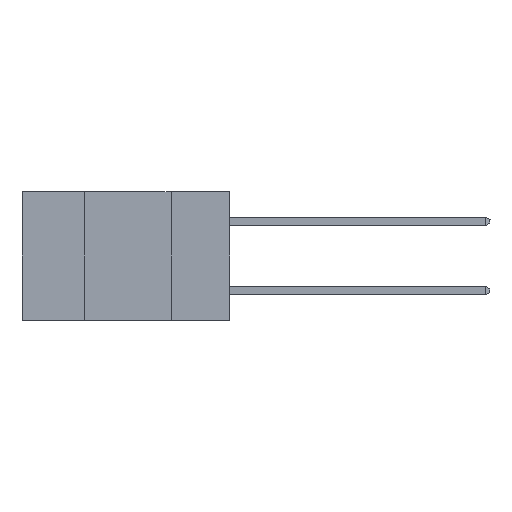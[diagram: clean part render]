
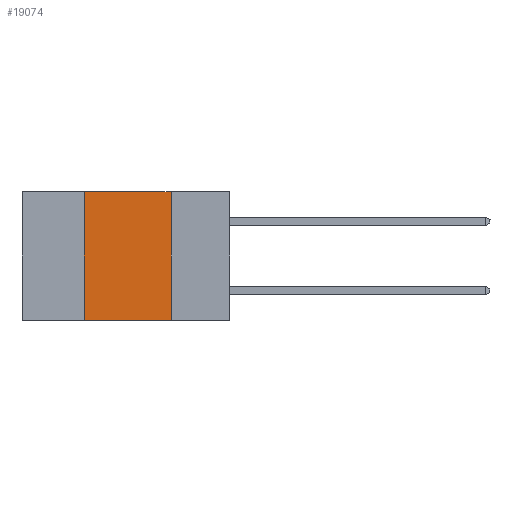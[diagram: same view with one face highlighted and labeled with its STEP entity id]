
A CAD part, left-side view. The second image highlights one B-rep face of the part: STEP entity #19074.
In plain terms, the highlighted planar face has unit normal (-1, 0, 0).
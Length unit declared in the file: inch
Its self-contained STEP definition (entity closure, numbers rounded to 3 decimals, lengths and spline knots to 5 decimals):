
#712 = DIRECTION ( 'NONE',  ( 0., 0., 1. ) ) ;
#1562 = CARTESIAN_POINT ( 'NONE',  ( 0., 0.17, -0.37 ) ) ;
#2390 = DIRECTION ( 'NONE',  ( 1., 0., 0. ) ) ;
#2484 = AXIS2_PLACEMENT_3D ( 'NONE', #10605, #2390, #7268 ) ;
#2840 = DIRECTION ( 'NONE',  ( 0., 0., -1. ) ) ;
#3261 = FACE_OUTER_BOUND ( 'NONE', #5779, .T. ) ;
#4365 = LINE ( 'NONE', #19323, #12798 ) ;
#4702 = VERTEX_POINT ( 'NONE', #7993 ) ;
#5711 = ORIENTED_EDGE ( 'NONE', *, *, #17642, .F. ) ;
#5779 = EDGE_LOOP ( 'NONE', ( #19456, #19666, #5711, #13531 ) ) ;
#5989 = VERTEX_POINT ( 'NONE', #1562 ) ;
#6096 = EDGE_CURVE ( 'NONE', #18754, #5989, #4365, .T. ) ;
#6382 = VECTOR ( 'NONE', #18672, 39.37008 ) ;
#6488 = CARTESIAN_POINT ( 'NONE',  ( 0., 0.17, 0. ) ) ;
#7091 = DIRECTION ( 'NONE',  ( 0., -1., 0. ) ) ;
#7180 = LINE ( 'NONE', #10670, #13827 ) ;
#7268 = DIRECTION ( 'NONE',  ( 0., 0., -1. ) ) ;
#7638 = CARTESIAN_POINT ( 'NONE',  ( 0., 0.42, 0. ) ) ;
#7993 = CARTESIAN_POINT ( 'NONE',  ( 0., 0.42, -0.37 ) ) ;
#8886 = PLANE ( 'NONE',  #2484 ) ;
#10605 = CARTESIAN_POINT ( 'NONE',  ( 0., 0.6, 0. ) ) ;
#10670 = CARTESIAN_POINT ( 'NONE',  ( 0., 0.42, 0. ) ) ;
#11717 = EDGE_CURVE ( 'NONE', #4702, #5989, #19223, .T. ) ;
#12798 = VECTOR ( 'NONE', #2840, 39.37008 ) ;
#13531 = ORIENTED_EDGE ( 'NONE', *, *, #11717, .T. ) ;
#13827 = VECTOR ( 'NONE', #712, 39.37008 ) ;
#14036 = CARTESIAN_POINT ( 'NONE',  ( 0., 0.6, 0. ) ) ;
#15431 = CARTESIAN_POINT ( 'NONE',  ( 0., 0.6, -0.37 ) ) ;
#16033 = LINE ( 'NONE', #14036, #18879 ) ;
#17642 = EDGE_CURVE ( 'NONE', #4702, #17789, #7180, .T. ) ;
#17789 = VERTEX_POINT ( 'NONE', #7638 ) ;
#18672 = DIRECTION ( 'NONE',  ( 0., -1., 0. ) ) ;
#18754 = VERTEX_POINT ( 'NONE', #6488 ) ;
#18879 = VECTOR ( 'NONE', #7091, 39.37008 ) ;
#19074 = ADVANCED_FACE ( 'NONE', ( #3261 ), #8886, .F. ) ;
#19223 = LINE ( 'NONE', #15431, #6382 ) ;
#19323 = CARTESIAN_POINT ( 'NONE',  ( 0., 0.17, 0. ) ) ;
#19456 = ORIENTED_EDGE ( 'NONE', *, *, #6096, .F. ) ;
#19666 = ORIENTED_EDGE ( 'NONE', *, *, #20920, .F. ) ;
#20920 = EDGE_CURVE ( 'NONE', #17789, #18754, #16033, .T. ) ;
